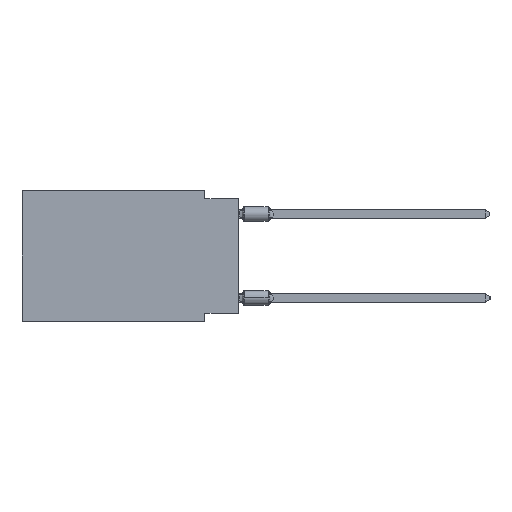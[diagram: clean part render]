
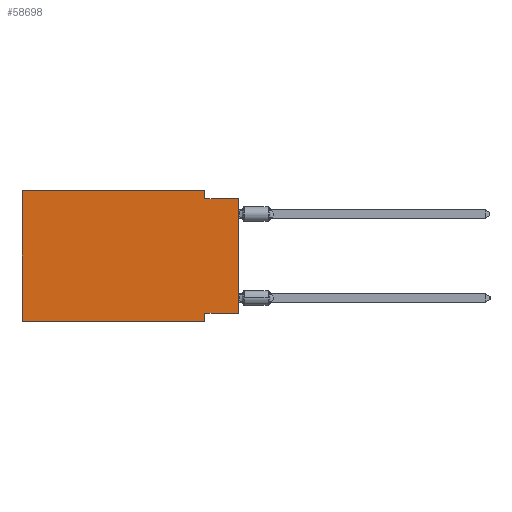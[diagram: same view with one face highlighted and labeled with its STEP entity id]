
A CAD part, left-side view. The second image highlights one B-rep face of the part: STEP entity #58698.
In plain terms, the highlighted planar face has unit normal (-1, 0, 0).
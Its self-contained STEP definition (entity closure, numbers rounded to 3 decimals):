
#221 = AXIS2_PLACEMENT_3D ( 'NONE', #7719, #61612, #23416 ) ;
#1637 = EDGE_CURVE ( 'NONE', #28913, #21110, #10893, .T. ) ;
#3061 = VECTOR ( 'NONE', #27085, 1000. ) ;
#4876 = CARTESIAN_POINT ( 'NONE',  ( 0., 16.383, 0. ) ) ;
#5183 = LINE ( 'NONE', #39829, #37506 ) ;
#5869 = VERTEX_POINT ( 'NONE', #36894 ) ;
#7209 = EDGE_LOOP ( 'NONE', ( #55358, #37883, #42919, #59903, #11797, #56747, #27389, #50239 ) ) ;
#7608 = EDGE_CURVE ( 'NONE', #27639, #27325, #63241, .T. ) ;
#7719 = CARTESIAN_POINT ( 'NONE',  ( 0., 16.383, 0. ) ) ;
#7988 = CARTESIAN_POINT ( 'NONE',  ( 0., 2.54, 0. ) ) ;
#8202 = CARTESIAN_POINT ( 'NONE',  ( 0., 0., -0.635 ) ) ;
#9531 = VERTEX_POINT ( 'NONE', #43572 ) ;
#9809 = VERTEX_POINT ( 'NONE', #8202 ) ;
#9990 = DIRECTION ( 'NONE',  ( 0., 0., 1. ) ) ;
#10573 = DIRECTION ( 'NONE',  ( 0., 1., 0. ) ) ;
#10893 = LINE ( 'NONE', #44926, #30376 ) ;
#11295 = VECTOR ( 'NONE', #9990, 1000. ) ;
#11797 = ORIENTED_EDGE ( 'NONE', *, *, #7608, .F. ) ;
#14396 = LINE ( 'NONE', #54818, #47055 ) ;
#17264 = CARTESIAN_POINT ( 'NONE',  ( 0., 2.54, -9.906 ) ) ;
#17400 = EDGE_CURVE ( 'NONE', #27325, #5869, #26779, .T. ) ;
#20897 = CARTESIAN_POINT ( 'NONE',  ( 0., 2.54, -9.271 ) ) ;
#21110 = VERTEX_POINT ( 'NONE', #20897 ) ;
#21115 = VECTOR ( 'NONE', #27566, 1000. ) ;
#22393 = LINE ( 'NONE', #57040, #23790 ) ;
#22714 = DIRECTION ( 'NONE',  ( 0., -1., 0. ) ) ;
#23416 = DIRECTION ( 'NONE',  ( 0., 0., -1. ) ) ;
#23790 = VECTOR ( 'NONE', #22714, 1000. ) ;
#24741 = DIRECTION ( 'NONE',  ( 0., -1., 0. ) ) ;
#26568 = EDGE_CURVE ( 'NONE', #5869, #9531, #32709, .T. ) ;
#26779 = LINE ( 'NONE', #46365, #3061 ) ;
#26814 = VECTOR ( 'NONE', #61108, 1000. ) ;
#27085 = DIRECTION ( 'NONE',  ( 0., -1., 0. ) ) ;
#27325 = VERTEX_POINT ( 'NONE', #49931 ) ;
#27389 = ORIENTED_EDGE ( 'NONE', *, *, #35427, .F. ) ;
#27566 = DIRECTION ( 'NONE',  ( 0., 0., -1. ) ) ;
#27639 = VERTEX_POINT ( 'NONE', #34142 ) ;
#28913 = VERTEX_POINT ( 'NONE', #45369 ) ;
#30376 = VECTOR ( 'NONE', #10573, 1000. ) ;
#31919 = EDGE_CURVE ( 'NONE', #27639, #43483, #5183, .T. ) ;
#32709 = LINE ( 'NONE', #7988, #21115 ) ;
#34142 = CARTESIAN_POINT ( 'NONE',  ( 0., 16.383, -9.906 ) ) ;
#35427 = EDGE_CURVE ( 'NONE', #21110, #43483, #14396, .T. ) ;
#36894 = CARTESIAN_POINT ( 'NONE',  ( 0., 2.54, 0. ) ) ;
#37506 = VECTOR ( 'NONE', #24741, 1000. ) ;
#37883 = ORIENTED_EDGE ( 'NONE', *, *, #59045, .F. ) ;
#39441 = DIRECTION ( 'NONE',  ( 0., 0., -1. ) ) ;
#39829 = CARTESIAN_POINT ( 'NONE',  ( 0., 16.383, -9.906 ) ) ;
#41554 = CARTESIAN_POINT ( 'NONE',  ( 0., 0., 0. ) ) ;
#42919 = ORIENTED_EDGE ( 'NONE', *, *, #26568, .F. ) ;
#43483 = VERTEX_POINT ( 'NONE', #17264 ) ;
#43572 = CARTESIAN_POINT ( 'NONE',  ( 0., 2.54, -0.635 ) ) ;
#44926 = CARTESIAN_POINT ( 'NONE',  ( 0., 0., -9.271 ) ) ;
#45369 = CARTESIAN_POINT ( 'NONE',  ( 0., 0., -9.271 ) ) ;
#46365 = CARTESIAN_POINT ( 'NONE',  ( 0., 16.383, 0. ) ) ;
#46687 = LINE ( 'NONE', #41554, #26814 ) ;
#47055 = VECTOR ( 'NONE', #39441, 1000. ) ;
#49061 = EDGE_CURVE ( 'NONE', #28913, #9809, #46687, .T. ) ;
#49931 = CARTESIAN_POINT ( 'NONE',  ( 0., 16.383, 0. ) ) ;
#50239 = ORIENTED_EDGE ( 'NONE', *, *, #1637, .F. ) ;
#52000 = PLANE ( 'NONE',  #221 ) ;
#54818 = CARTESIAN_POINT ( 'NONE',  ( 0., 2.54, -9.906 ) ) ;
#55358 = ORIENTED_EDGE ( 'NONE', *, *, #49061, .T. ) ;
#56747 = ORIENTED_EDGE ( 'NONE', *, *, #31919, .T. ) ;
#56799 = FACE_OUTER_BOUND ( 'NONE', #7209, .T. ) ;
#57040 = CARTESIAN_POINT ( 'NONE',  ( 0., 0., -0.635 ) ) ;
#58698 = ADVANCED_FACE ( 'NONE', ( #56799 ), #52000, .F. ) ;
#59045 = EDGE_CURVE ( 'NONE', #9531, #9809, #22393, .T. ) ;
#59903 = ORIENTED_EDGE ( 'NONE', *, *, #17400, .F. ) ;
#61108 = DIRECTION ( 'NONE',  ( 0., 0., 1. ) ) ;
#61612 = DIRECTION ( 'NONE',  ( 1., 0., 0. ) ) ;
#63241 = LINE ( 'NONE', #4876, #11295 ) ;
